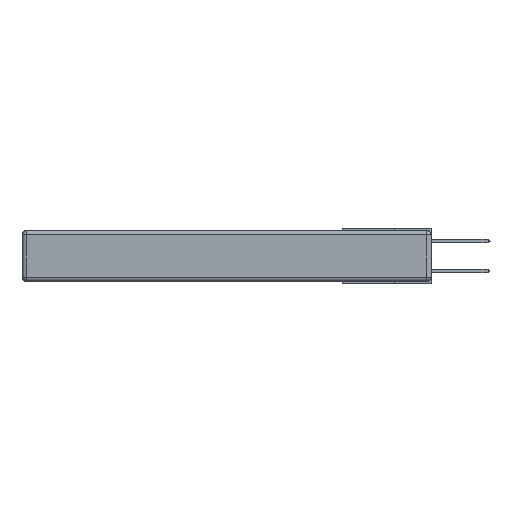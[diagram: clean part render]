
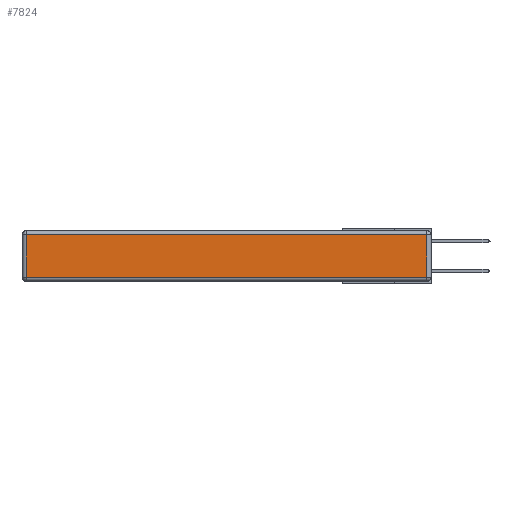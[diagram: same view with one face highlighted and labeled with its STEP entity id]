
A CAD part, left-side view. The second image highlights one B-rep face of the part: STEP entity #7824.
In plain terms, the highlighted planar face has unit normal (-1, 0, 0).
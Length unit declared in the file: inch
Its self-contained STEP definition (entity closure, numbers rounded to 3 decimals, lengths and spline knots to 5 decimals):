
#439 = LINE ( 'NONE', #15280, #4251 ) ;
#664 = FACE_OUTER_BOUND ( 'NONE', #11881, .T. ) ;
#1005 = EDGE_CURVE ( 'NONE', #13295, #18564, #11887, .T. ) ;
#1262 = ORIENTED_EDGE ( 'NONE', *, *, #1005, .T. ) ;
#1793 = DIRECTION ( 'NONE',  ( 0., -1., 0. ) ) ;
#2566 = CARTESIAN_POINT ( 'NONE',  ( 0., 2.72, -0.313 ) ) ;
#2684 = CARTESIAN_POINT ( 'NONE',  ( 0., 0.03, -0.313 ) ) ;
#3405 = DIRECTION ( 'NONE',  ( 0., 0., 1. ) ) ;
#3699 = DIRECTION ( 'NONE',  ( 0., 1., 0. ) ) ;
#4251 = VECTOR ( 'NONE', #3405, 39.37008 ) ;
#4667 = CARTESIAN_POINT ( 'NONE',  ( 0., 2.72, -0.03 ) ) ;
#5162 = VECTOR ( 'NONE', #3699, 39.37008 ) ;
#5350 = VERTEX_POINT ( 'NONE', #2566 ) ;
#7485 = LINE ( 'NONE', #16992, #16334 ) ;
#7824 = ADVANCED_FACE ( 'NONE', ( #664 ), #12192, .T. ) ;
#9817 = EDGE_CURVE ( 'NONE', #15719, #13295, #439, .T. ) ;
#9830 = CARTESIAN_POINT ( 'NONE',  ( 0., 0.03, -0.03 ) ) ;
#11535 = ORIENTED_EDGE ( 'NONE', *, *, #9817, .T. ) ;
#11881 = EDGE_LOOP ( 'NONE', ( #13991, #11535, #1262, #15436 ) ) ;
#11887 = LINE ( 'NONE', #12870, #5162 ) ;
#12192 = PLANE ( 'NONE',  #17002 ) ;
#12255 = DIRECTION ( 'NONE',  ( -1., 0., 0. ) ) ;
#12444 = CARTESIAN_POINT ( 'NONE',  ( 0., 0., -0.313 ) ) ;
#12870 = CARTESIAN_POINT ( 'NONE',  ( 0., 2.75, -0.03 ) ) ;
#13295 = VERTEX_POINT ( 'NONE', #9830 ) ;
#13460 = EDGE_CURVE ( 'NONE', #18564, #5350, #7485, .T. ) ;
#13794 = DIRECTION ( 'NONE',  ( 0., 0., 1. ) ) ;
#13991 = ORIENTED_EDGE ( 'NONE', *, *, #16762, .T. ) ;
#14051 = DIRECTION ( 'NONE',  ( 0., 0., -1. ) ) ;
#14118 = LINE ( 'NONE', #12444, #17001 ) ;
#15280 = CARTESIAN_POINT ( 'NONE',  ( 0., 0.03, -0.343 ) ) ;
#15436 = ORIENTED_EDGE ( 'NONE', *, *, #13460, .T. ) ;
#15719 = VERTEX_POINT ( 'NONE', #2684 ) ;
#16334 = VECTOR ( 'NONE', #14051, 39.37008 ) ;
#16762 = EDGE_CURVE ( 'NONE', #5350, #15719, #14118, .T. ) ;
#16992 = CARTESIAN_POINT ( 'NONE',  ( 0., 2.72, -0.343 ) ) ;
#17001 = VECTOR ( 'NONE', #1793, 39.37008 ) ;
#17002 = AXIS2_PLACEMENT_3D ( 'NONE', #18354, #12255, #13794 ) ;
#18354 = CARTESIAN_POINT ( 'NONE',  ( 0., 0., -0.343 ) ) ;
#18564 = VERTEX_POINT ( 'NONE', #4667 ) ;
